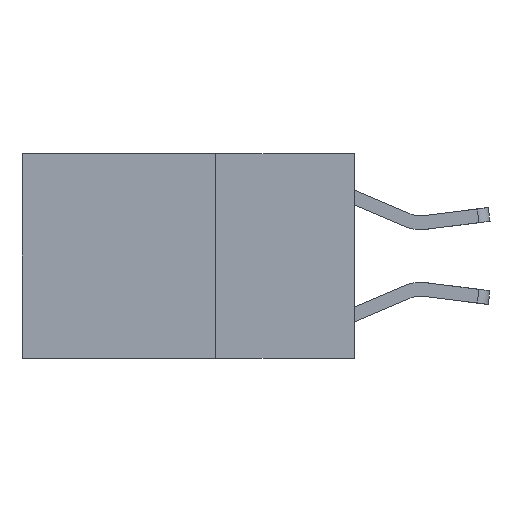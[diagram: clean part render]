
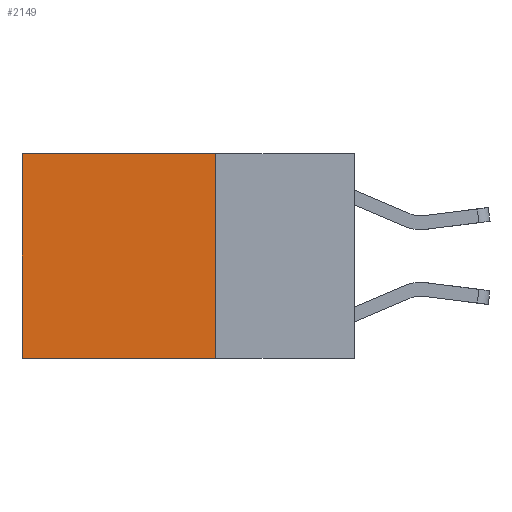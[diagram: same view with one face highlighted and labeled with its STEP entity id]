
A CAD part, left-side view. The second image highlights one B-rep face of the part: STEP entity #2149.
In plain terms, the highlighted planar face has unit normal (-1, 0, 0).
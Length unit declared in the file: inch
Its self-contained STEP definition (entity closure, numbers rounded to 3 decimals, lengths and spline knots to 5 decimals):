
#997 = CARTESIAN_POINT ( 'NONE',  ( 0.2625, 0.25, -0.37 ) ) ;
#1219 = LINE ( 'NONE', #10396, #3481 ) ;
#1356 = VECTOR ( 'NONE', #6106, 39.37008 ) ;
#1484 = ORIENTED_EDGE ( 'NONE', *, *, #3444, .T. ) ;
#2149 = ADVANCED_FACE ( 'NONE', ( #7228 ), #6179, .F. ) ;
#2311 = VECTOR ( 'NONE', #10583, 39.37008 ) ;
#2314 = EDGE_CURVE ( 'NONE', #4106, #5901, #3634, .T. ) ;
#2368 = VERTEX_POINT ( 'NONE', #5754 ) ;
#2554 = CARTESIAN_POINT ( 'NONE',  ( 0.2625, 0.25, 0. ) ) ;
#3132 = CARTESIAN_POINT ( 'NONE',  ( 0.2625, 0.25, 0. ) ) ;
#3444 = EDGE_CURVE ( 'NONE', #2368, #6772, #1219, .T. ) ;
#3481 = VECTOR ( 'NONE', #3621, 39.37008 ) ;
#3621 = DIRECTION ( 'NONE',  ( 0., 0., -1. ) ) ;
#3634 = LINE ( 'NONE', #3132, #2311 ) ;
#4104 = AXIS2_PLACEMENT_3D ( 'NONE', #8776, #7890, #6216 ) ;
#4106 = VERTEX_POINT ( 'NONE', #2554 ) ;
#4167 = EDGE_LOOP ( 'NONE', ( #1484, #9648, #7839, #6994 ) ) ;
#4235 = CARTESIAN_POINT ( 'NONE',  ( 0.2625, 0.25, -0.37 ) ) ;
#5564 = EDGE_CURVE ( 'NONE', #5901, #6772, #5681, .T. ) ;
#5681 = LINE ( 'NONE', #4235, #9075 ) ;
#5754 = CARTESIAN_POINT ( 'NONE',  ( 0.2625, 0.6, 0. ) ) ;
#5901 = VERTEX_POINT ( 'NONE', #997 ) ;
#6106 = DIRECTION ( 'NONE',  ( 0., 1., 0. ) ) ;
#6179 = PLANE ( 'NONE',  #4104 ) ;
#6216 = DIRECTION ( 'NONE',  ( 0., 0., -1. ) ) ;
#6714 = DIRECTION ( 'NONE',  ( 0., 1., 0. ) ) ;
#6771 = EDGE_CURVE ( 'NONE', #4106, #2368, #10594, .T. ) ;
#6772 = VERTEX_POINT ( 'NONE', #9518 ) ;
#6994 = ORIENTED_EDGE ( 'NONE', *, *, #6771, .T. ) ;
#7228 = FACE_OUTER_BOUND ( 'NONE', #4167, .T. ) ;
#7839 = ORIENTED_EDGE ( 'NONE', *, *, #2314, .F. ) ;
#7851 = CARTESIAN_POINT ( 'NONE',  ( 0.2625, 0.25, 0. ) ) ;
#7890 = DIRECTION ( 'NONE',  ( 1., 0., 0. ) ) ;
#8776 = CARTESIAN_POINT ( 'NONE',  ( 0.2625, 0.25, 0. ) ) ;
#9075 = VECTOR ( 'NONE', #6714, 39.37008 ) ;
#9518 = CARTESIAN_POINT ( 'NONE',  ( 0.2625, 0.6, -0.37 ) ) ;
#9648 = ORIENTED_EDGE ( 'NONE', *, *, #5564, .F. ) ;
#10396 = CARTESIAN_POINT ( 'NONE',  ( 0.2625, 0.6, 0. ) ) ;
#10583 = DIRECTION ( 'NONE',  ( 0., 0., -1. ) ) ;
#10594 = LINE ( 'NONE', #7851, #1356 ) ;
